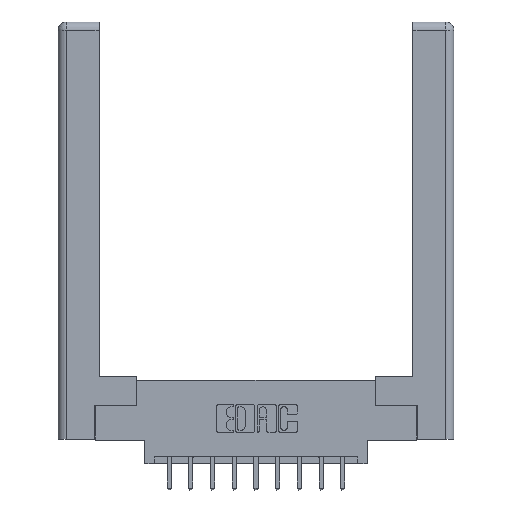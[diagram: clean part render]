
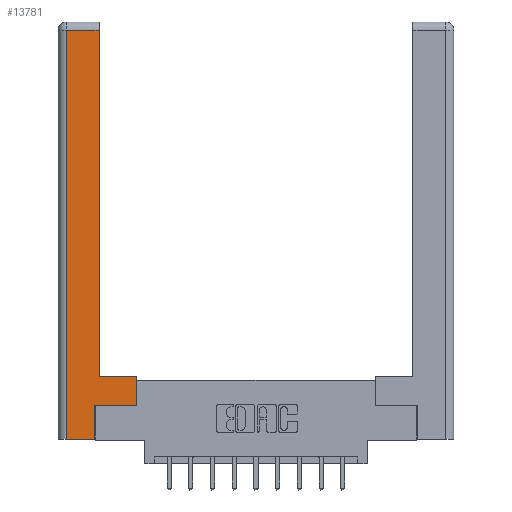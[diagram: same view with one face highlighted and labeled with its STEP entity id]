
A CAD part, top view. The second image highlights one B-rep face of the part: STEP entity #13781.
In plain terms, the highlighted planar face has unit normal (0, 0, 1).
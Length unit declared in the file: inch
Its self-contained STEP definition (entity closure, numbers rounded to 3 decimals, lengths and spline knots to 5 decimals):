
#169 = CARTESIAN_POINT ( 'NONE',  ( 0.565, 0.245, 0. ) ) ;
#225 = ORIENTED_EDGE ( 'NONE', *, *, #13957, .T. ) ;
#363 = FACE_OUTER_BOUND ( 'NONE', #3064, .T. ) ;
#1835 = VERTEX_POINT ( 'NONE', #8870 ) ;
#1869 = LINE ( 'NONE', #5779, #12833 ) ;
#2375 = DIRECTION ( 'NONE',  ( 1., 0., 0. ) ) ;
#2795 = VERTEX_POINT ( 'NONE', #6463 ) ;
#2872 = DIRECTION ( 'NONE',  ( 0., 1., 0. ) ) ;
#3064 = EDGE_LOOP ( 'NONE', ( #3421, #5320, #13853, #13341, #225, #12970, #11663, #3303 ) ) ;
#3121 = LINE ( 'NONE', #169, #3642 ) ;
#3303 = ORIENTED_EDGE ( 'NONE', *, *, #4645, .T. ) ;
#3367 = AXIS2_PLACEMENT_3D ( 'NONE', #6311, #12760, #6210 ) ;
#3421 = ORIENTED_EDGE ( 'NONE', *, *, #5876, .T. ) ;
#3422 = CARTESIAN_POINT ( 'NONE',  ( 0.565, 0.245, 0. ) ) ;
#3642 = VECTOR ( 'NONE', #2375, 39.37008 ) ;
#3709 = EDGE_CURVE ( 'NONE', #12615, #10894, #8986, .T. ) ;
#3924 = VECTOR ( 'NONE', #8575, 39.37008 ) ;
#4423 = CARTESIAN_POINT ( 'NONE',  ( 0.265, 0., 0. ) ) ;
#4494 = LINE ( 'NONE', #9890, #13885 ) ;
#4614 = LINE ( 'NONE', #4423, #3924 ) ;
#4645 = EDGE_CURVE ( 'NONE', #10894, #10337, #11203, .T. ) ;
#4822 = LINE ( 'NONE', #12779, #10115 ) ;
#5229 = VERTEX_POINT ( 'NONE', #14095 ) ;
#5290 = CARTESIAN_POINT ( 'NONE',  ( 0.565, 0.45, 0. ) ) ;
#5320 = ORIENTED_EDGE ( 'NONE', *, *, #13335, .T. ) ;
#5779 = CARTESIAN_POINT ( 'NONE',  ( 0.0615, 0., 0. ) ) ;
#5876 = EDGE_CURVE ( 'NONE', #10337, #10639, #8584, .T. ) ;
#6079 = EDGE_CURVE ( 'NONE', #2795, #12615, #3121, .T. ) ;
#6210 = DIRECTION ( 'NONE',  ( -1., 0., 0. ) ) ;
#6212 = VECTOR ( 'NONE', #14078, 39.37008 ) ;
#6311 = CARTESIAN_POINT ( 'NONE',  ( 0., 0., 0. ) ) ;
#6463 = CARTESIAN_POINT ( 'NONE',  ( 0.265, 0.245, 0. ) ) ;
#6712 = DIRECTION ( 'NONE',  ( -1., 0., 0. ) ) ;
#7263 = CARTESIAN_POINT ( 'NONE',  ( 0.295, 0.45, 0. ) ) ;
#7382 = PLANE ( 'NONE',  #3367 ) ;
#7755 = CARTESIAN_POINT ( 'NONE',  ( 0.295, 0.45, 0. ) ) ;
#8011 = CARTESIAN_POINT ( 'NONE',  ( 0.565, 0.45, 0. ) ) ;
#8289 = VECTOR ( 'NONE', #10554, 39.37008 ) ;
#8575 = DIRECTION ( 'NONE',  ( 1., 0., 0. ) ) ;
#8584 = LINE ( 'NONE', #12995, #6212 ) ;
#8870 = CARTESIAN_POINT ( 'NONE',  ( 0.265, 0., 0. ) ) ;
#8986 = LINE ( 'NONE', #8011, #11923 ) ;
#9062 = EDGE_CURVE ( 'NONE', #5229, #12621, #1869, .T. ) ;
#9089 = DIRECTION ( 'NONE',  ( 0., 1., 0. ) ) ;
#9365 = EDGE_CURVE ( 'NONE', #12621, #1835, #4614, .T. ) ;
#9890 = CARTESIAN_POINT ( 'NONE',  ( 0.0615, 2.94, 0. ) ) ;
#10115 = VECTOR ( 'NONE', #2872, 39.37008 ) ;
#10337 = VERTEX_POINT ( 'NONE', #7755 ) ;
#10554 = DIRECTION ( 'NONE',  ( -1., 0., 0. ) ) ;
#10639 = VERTEX_POINT ( 'NONE', #12784 ) ;
#10894 = VERTEX_POINT ( 'NONE', #5290 ) ;
#11203 = LINE ( 'NONE', #7263, #8289 ) ;
#11663 = ORIENTED_EDGE ( 'NONE', *, *, #3709, .T. ) ;
#11923 = VECTOR ( 'NONE', #9089, 39.37008 ) ;
#12173 = DIRECTION ( 'NONE',  ( 0., -1., 0. ) ) ;
#12182 = CARTESIAN_POINT ( 'NONE',  ( 0.0615, 0., 0. ) ) ;
#12615 = VERTEX_POINT ( 'NONE', #3422 ) ;
#12621 = VERTEX_POINT ( 'NONE', #12182 ) ;
#12760 = DIRECTION ( 'NONE',  ( 0., 0., -1. ) ) ;
#12779 = CARTESIAN_POINT ( 'NONE',  ( 0.265, 0.245, 0. ) ) ;
#12784 = CARTESIAN_POINT ( 'NONE',  ( 0.295, 2.94, 0. ) ) ;
#12833 = VECTOR ( 'NONE', #12173, 39.37008 ) ;
#12970 = ORIENTED_EDGE ( 'NONE', *, *, #6079, .T. ) ;
#12995 = CARTESIAN_POINT ( 'NONE',  ( 0.295, 3., 0. ) ) ;
#13335 = EDGE_CURVE ( 'NONE', #10639, #5229, #4494, .T. ) ;
#13341 = ORIENTED_EDGE ( 'NONE', *, *, #9365, .T. ) ;
#13781 = ADVANCED_FACE ( 'NONE', ( #363 ), #7382, .F. ) ;
#13853 = ORIENTED_EDGE ( 'NONE', *, *, #9062, .T. ) ;
#13885 = VECTOR ( 'NONE', #6712, 39.37008 ) ;
#13957 = EDGE_CURVE ( 'NONE', #1835, #2795, #4822, .T. ) ;
#14078 = DIRECTION ( 'NONE',  ( 0., 1., 0. ) ) ;
#14095 = CARTESIAN_POINT ( 'NONE',  ( 0.0615, 2.94, 0. ) ) ;
